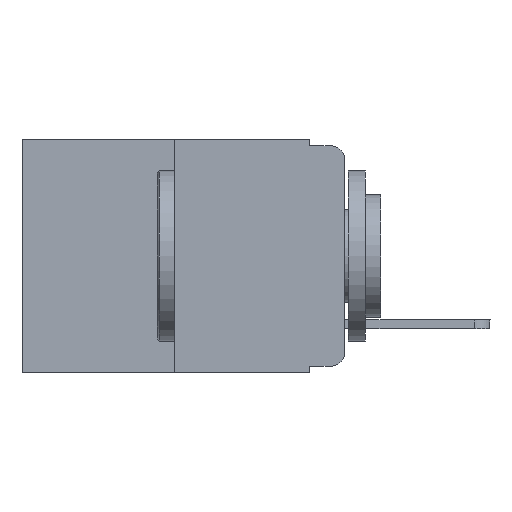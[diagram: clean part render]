
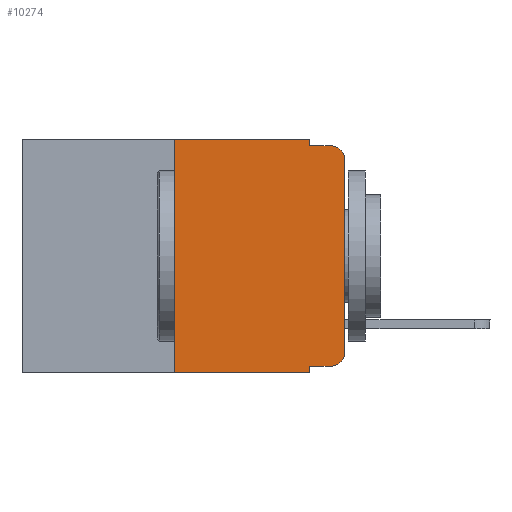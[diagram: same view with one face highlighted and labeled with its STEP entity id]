
A CAD part, left-side view. The second image highlights one B-rep face of the part: STEP entity #10274.
In plain terms, the highlighted planar face has unit normal (-1, 0, 0).
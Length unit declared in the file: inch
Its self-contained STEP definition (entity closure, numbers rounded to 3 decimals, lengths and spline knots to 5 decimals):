
#14 = CARTESIAN_POINT ( 'NONE',  ( 0., 0.051, -0.01 ) ) ;
#253 = LINE ( 'NONE', #6975, #7379 ) ;
#349 = ORIENTED_EDGE ( 'NONE', *, *, #4358, .F. ) ;
#731 = ORIENTED_EDGE ( 'NONE', *, *, #4835, .F. ) ;
#847 = EDGE_CURVE ( 'NONE', #8434, #5040, #8321, .T. ) ;
#1093 = VECTOR ( 'NONE', #6972, 39.37008 ) ;
#1183 = CARTESIAN_POINT ( 'NONE',  ( 0., 0.473, 0. ) ) ;
#1389 = VERTEX_POINT ( 'NONE', #8262 ) ;
#1446 = DIRECTION ( 'NONE',  ( 0., 0., -1. ) ) ;
#1709 = AXIS2_PLACEMENT_3D ( 'NONE', #11346, #12065, #9335 ) ;
#2408 = DIRECTION ( 'NONE',  ( 0., 0., -1. ) ) ;
#2480 = EDGE_CURVE ( 'NONE', #3488, #4765, #10732, .T. ) ;
#2496 = VECTOR ( 'NONE', #10752, 39.37008 ) ;
#2526 = LINE ( 'NONE', #6120, #1093 ) ;
#2638 = EDGE_CURVE ( 'NONE', #11267, #5498, #2526, .T. ) ;
#2678 = VERTEX_POINT ( 'NONE', #4200 ) ;
#2817 = DIRECTION ( 'NONE',  ( 0., -1., 0. ) ) ;
#2943 = ORIENTED_EDGE ( 'NONE', *, *, #2638, .T. ) ;
#3178 = EDGE_CURVE ( 'NONE', #4765, #3661, #11865, .T. ) ;
#3191 = LINE ( 'NONE', #7094, #9789 ) ;
#3243 = VECTOR ( 'NONE', #10518, 39.37008 ) ;
#3366 = CARTESIAN_POINT ( 'NONE',  ( 0., 0.051, 0. ) ) ;
#3488 = VERTEX_POINT ( 'NONE', #6511 ) ;
#3552 = VERTEX_POINT ( 'NONE', #5686 ) ;
#3661 = VERTEX_POINT ( 'NONE', #4940 ) ;
#3724 = EDGE_CURVE ( 'NONE', #11267, #1389, #4948, .T. ) ;
#4000 = LINE ( 'NONE', #14, #7366 ) ;
#4090 = CARTESIAN_POINT ( 'NONE',  ( 0., 0.051, 0. ) ) ;
#4200 = CARTESIAN_POINT ( 'NONE',  ( 0., 0.25, -0.343 ) ) ;
#4269 = DIRECTION ( 'NONE',  ( 0., -1., 0. ) ) ;
#4358 = EDGE_CURVE ( 'NONE', #2678, #3488, #253, .T. ) ;
#4380 = EDGE_LOOP ( 'NONE', ( #6386, #7160, #731, #8240, #5989, #349, #5392, #8145, #2943, #10355 ) ) ;
#4515 = CIRCLE ( 'NONE', #6281, 0.02 ) ;
#4765 = VERTEX_POINT ( 'NONE', #3366 ) ;
#4835 = EDGE_CURVE ( 'NONE', #3661, #3552, #4000, .T. ) ;
#4940 = CARTESIAN_POINT ( 'NONE',  ( 0., 0.051, -0.01 ) ) ;
#4948 = LINE ( 'NONE', #4090, #2496 ) ;
#5040 = VERTEX_POINT ( 'NONE', #8888 ) ;
#5230 = FACE_OUTER_BOUND ( 'NONE', #4380, .T. ) ;
#5392 = ORIENTED_EDGE ( 'NONE', *, *, #9272, .T. ) ;
#5498 = VERTEX_POINT ( 'NONE', #11863 ) ;
#5538 = CIRCLE ( 'NONE', #6118, 0.02 ) ;
#5686 = CARTESIAN_POINT ( 'NONE',  ( 0., 0.02, -0.01 ) ) ;
#5809 = VECTOR ( 'NONE', #10626, 39.37008 ) ;
#5950 = CARTESIAN_POINT ( 'NONE',  ( 0., 0.051, -0.333 ) ) ;
#5989 = ORIENTED_EDGE ( 'NONE', *, *, #2480, .F. ) ;
#6019 = CARTESIAN_POINT ( 'NONE',  ( 0., 0.02, -0.313 ) ) ;
#6118 = AXIS2_PLACEMENT_3D ( 'NONE', #6019, #11771, #1446 ) ;
#6120 = CARTESIAN_POINT ( 'NONE',  ( 0., 0.051, -0.333 ) ) ;
#6281 = AXIS2_PLACEMENT_3D ( 'NONE', #6990, #7999, #2408 ) ;
#6386 = ORIENTED_EDGE ( 'NONE', *, *, #847, .T. ) ;
#6511 = CARTESIAN_POINT ( 'NONE',  ( 0., 0.25, 0. ) ) ;
#6972 = DIRECTION ( 'NONE',  ( 0., -1., 0. ) ) ;
#6975 = CARTESIAN_POINT ( 'NONE',  ( 0., 0.25, 0. ) ) ;
#6990 = CARTESIAN_POINT ( 'NONE',  ( 0., 0.02, -0.03 ) ) ;
#7094 = CARTESIAN_POINT ( 'NONE',  ( 0., 0.473, -0.343 ) ) ;
#7160 = ORIENTED_EDGE ( 'NONE', *, *, #8731, .T. ) ;
#7366 = VECTOR ( 'NONE', #2817, 39.37008 ) ;
#7379 = VECTOR ( 'NONE', #11583, 39.37008 ) ;
#7454 = VECTOR ( 'NONE', #11606, 39.37008 ) ;
#7656 = CARTESIAN_POINT ( 'NONE',  ( 0., 0., 0. ) ) ;
#7999 = DIRECTION ( 'NONE',  ( -1., 0., 0. ) ) ;
#8145 = ORIENTED_EDGE ( 'NONE', *, *, #3724, .F. ) ;
#8240 = ORIENTED_EDGE ( 'NONE', *, *, #3178, .F. ) ;
#8262 = CARTESIAN_POINT ( 'NONE',  ( 0., 0.051, -0.343 ) ) ;
#8321 = LINE ( 'NONE', #7656, #5809 ) ;
#8434 = VERTEX_POINT ( 'NONE', #11285 ) ;
#8664 = EDGE_CURVE ( 'NONE', #5498, #8434, #5538, .T. ) ;
#8731 = EDGE_CURVE ( 'NONE', #5040, #3552, #4515, .T. ) ;
#8888 = CARTESIAN_POINT ( 'NONE',  ( 0., 0., -0.03 ) ) ;
#9272 = EDGE_CURVE ( 'NONE', #2678, #1389, #3191, .T. ) ;
#9335 = DIRECTION ( 'NONE',  ( 0., 0., -1. ) ) ;
#9416 = PLANE ( 'NONE',  #1709 ) ;
#9789 = VECTOR ( 'NONE', #4269, 39.37008 ) ;
#10274 = ADVANCED_FACE ( 'NONE', ( #5230 ), #9416, .F. ) ;
#10355 = ORIENTED_EDGE ( 'NONE', *, *, #8664, .T. ) ;
#10518 = DIRECTION ( 'NONE',  ( 0., -1., 0. ) ) ;
#10626 = DIRECTION ( 'NONE',  ( 0., 0., 1. ) ) ;
#10675 = CARTESIAN_POINT ( 'NONE',  ( 0., 0.051, 0. ) ) ;
#10732 = LINE ( 'NONE', #1183, #3243 ) ;
#10752 = DIRECTION ( 'NONE',  ( 0., 0., -1. ) ) ;
#11267 = VERTEX_POINT ( 'NONE', #5950 ) ;
#11285 = CARTESIAN_POINT ( 'NONE',  ( 0., 0., -0.313 ) ) ;
#11346 = CARTESIAN_POINT ( 'NONE',  ( 0., 0.473, 0. ) ) ;
#11583 = DIRECTION ( 'NONE',  ( 0., 0., 1. ) ) ;
#11606 = DIRECTION ( 'NONE',  ( 0., 0., -1. ) ) ;
#11771 = DIRECTION ( 'NONE',  ( -1., 0., 0. ) ) ;
#11863 = CARTESIAN_POINT ( 'NONE',  ( 0., 0.02, -0.333 ) ) ;
#11865 = LINE ( 'NONE', #10675, #7454 ) ;
#12065 = DIRECTION ( 'NONE',  ( 1., 0., 0. ) ) ;
